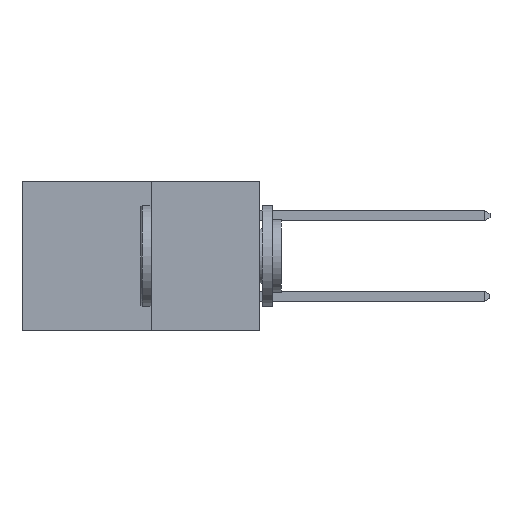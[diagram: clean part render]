
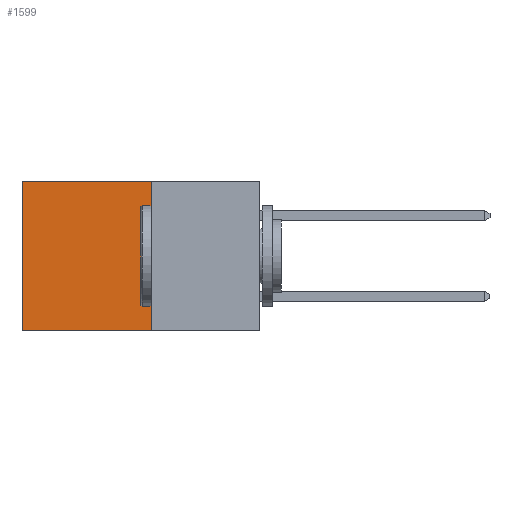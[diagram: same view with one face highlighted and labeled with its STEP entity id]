
A CAD part, left-side view. The second image highlights one B-rep face of the part: STEP entity #1599.
In plain terms, the highlighted planar face has unit normal (-1, 0, 0).
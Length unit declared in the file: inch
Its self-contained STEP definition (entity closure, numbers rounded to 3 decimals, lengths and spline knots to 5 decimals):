
#642 = FACE_OUTER_BOUND ( 'NONE', #4086, .T. ) ;
#1195 = CARTESIAN_POINT ( 'NONE',  ( 0.277, 0.59, 0. ) ) ;
#1599 = ADVANCED_FACE ( 'NONE', ( #642 ), #6233, .F. ) ;
#1742 = CARTESIAN_POINT ( 'NONE',  ( 0.277, 0.27, -0.37 ) ) ;
#1967 = ORIENTED_EDGE ( 'NONE', *, *, #5115, .T. ) ;
#2402 = DIRECTION ( 'NONE',  ( 0., 0., -1. ) ) ;
#2541 = VERTEX_POINT ( 'NONE', #6954 ) ;
#2902 = AXIS2_PLACEMENT_3D ( 'NONE', #6307, #6400, #6385 ) ;
#2942 = CARTESIAN_POINT ( 'NONE',  ( 0.277, 0.27, 0. ) ) ;
#3286 = CARTESIAN_POINT ( 'NONE',  ( 0.277, 0.27, -0.37 ) ) ;
#3602 = DIRECTION ( 'NONE',  ( 0., 1., 0. ) ) ;
#3757 = ORIENTED_EDGE ( 'NONE', *, *, #4483, .F. ) ;
#3992 = ORIENTED_EDGE ( 'NONE', *, *, #8283, .T. ) ;
#4086 = EDGE_LOOP ( 'NONE', ( #1967, #7825, #3757, #3992 ) ) ;
#4479 = LINE ( 'NONE', #3286, #7655 ) ;
#4483 = EDGE_CURVE ( 'NONE', #2541, #7504, #7668, .T. ) ;
#4990 = VECTOR ( 'NONE', #7744, 39.37008 ) ;
#5115 = EDGE_CURVE ( 'NONE', #5943, #5496, #5191, .T. ) ;
#5191 = LINE ( 'NONE', #7726, #4990 ) ;
#5278 = LINE ( 'NONE', #2942, #8402 ) ;
#5450 = CARTESIAN_POINT ( 'NONE',  ( 0.277, 0.59, -0.37 ) ) ;
#5496 = VERTEX_POINT ( 'NONE', #5450 ) ;
#5943 = VERTEX_POINT ( 'NONE', #1195 ) ;
#6003 = VECTOR ( 'NONE', #2402, 39.37008 ) ;
#6233 = PLANE ( 'NONE',  #2902 ) ;
#6307 = CARTESIAN_POINT ( 'NONE',  ( 0.277, 0.27, -0.37 ) ) ;
#6385 = DIRECTION ( 'NONE',  ( 0., 0., -1. ) ) ;
#6400 = DIRECTION ( 'NONE',  ( 1., 0., 0. ) ) ;
#6954 = CARTESIAN_POINT ( 'NONE',  ( 0.277, 0.27, 0. ) ) ;
#7504 = VERTEX_POINT ( 'NONE', #7553 ) ;
#7553 = CARTESIAN_POINT ( 'NONE',  ( 0.277, 0.27, -0.37 ) ) ;
#7655 = VECTOR ( 'NONE', #8385, 39.37008 ) ;
#7668 = LINE ( 'NONE', #1742, #6003 ) ;
#7726 = CARTESIAN_POINT ( 'NONE',  ( 0.277, 0.59, -0.37 ) ) ;
#7744 = DIRECTION ( 'NONE',  ( 0., 0., -1. ) ) ;
#7825 = ORIENTED_EDGE ( 'NONE', *, *, #7859, .F. ) ;
#7859 = EDGE_CURVE ( 'NONE', #7504, #5496, #4479, .T. ) ;
#8283 = EDGE_CURVE ( 'NONE', #2541, #5943, #5278, .T. ) ;
#8385 = DIRECTION ( 'NONE',  ( 0., 1., 0. ) ) ;
#8402 = VECTOR ( 'NONE', #3602, 39.37008 ) ;
